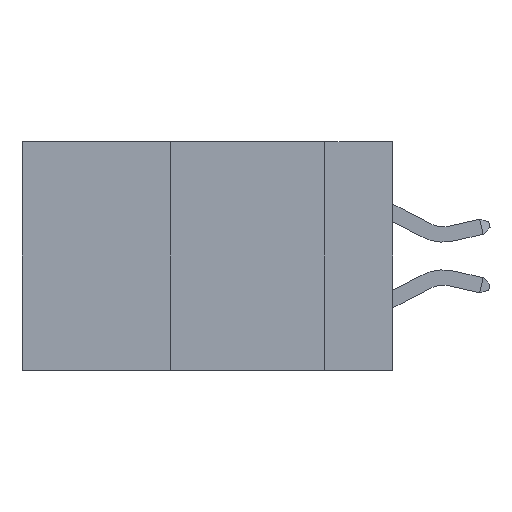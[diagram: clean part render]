
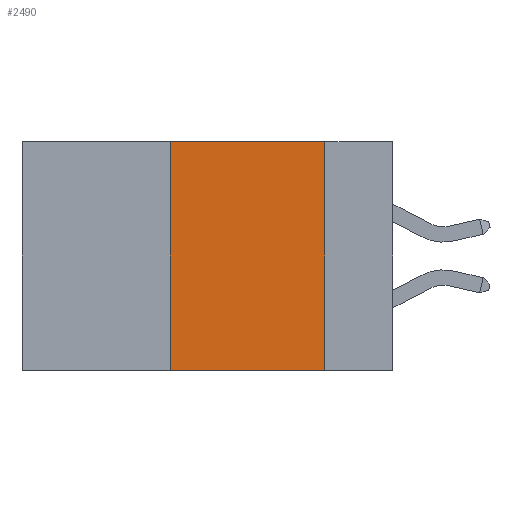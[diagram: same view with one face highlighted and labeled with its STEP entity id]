
A CAD part, left-side view. The second image highlights one B-rep face of the part: STEP entity #2490.
In plain terms, the highlighted planar face has unit normal (-1, 0, 0).
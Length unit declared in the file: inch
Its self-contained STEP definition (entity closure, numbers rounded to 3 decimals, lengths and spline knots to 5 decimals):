
#226 = ORIENTED_EDGE ( 'NONE', *, *, #5466, .F. ) ;
#1595 = VERTEX_POINT ( 'NONE', #4793 ) ;
#1841 = CARTESIAN_POINT ( 'NONE',  ( 0., 0.6, -0.37 ) ) ;
#2490 = ADVANCED_FACE ( 'NONE', ( #16931 ), #11524, .F. ) ;
#2787 = EDGE_LOOP ( 'NONE', ( #31848, #226, #22144, #26153 ) ) ;
#4539 = LINE ( 'NONE', #15166, #14033 ) ;
#4793 = CARTESIAN_POINT ( 'NONE',  ( 0., 0.11, -0.37 ) ) ;
#5466 = EDGE_CURVE ( 'NONE', #10425, #24842, #10987, .T. ) ;
#7572 = DIRECTION ( 'NONE',  ( 0., -1., 0. ) ) ;
#7695 = DIRECTION ( 'NONE',  ( 0., -1., 0. ) ) ;
#8708 = VECTOR ( 'NONE', #33378, 39.37008 ) ;
#9865 = CARTESIAN_POINT ( 'NONE',  ( 0., 0.11, 0. ) ) ;
#10425 = VERTEX_POINT ( 'NONE', #34082 ) ;
#10657 = VECTOR ( 'NONE', #7572, 39.37008 ) ;
#10987 = LINE ( 'NONE', #18673, #29775 ) ;
#11524 = PLANE ( 'NONE',  #22642 ) ;
#11632 = CARTESIAN_POINT ( 'NONE',  ( 0., 0.36, -0.37 ) ) ;
#13168 = EDGE_CURVE ( 'NONE', #21010, #10425, #4539, .T. ) ;
#13965 = DIRECTION ( 'NONE',  ( 0., 0., -1. ) ) ;
#14033 = VECTOR ( 'NONE', #25783, 39.37008 ) ;
#15166 = CARTESIAN_POINT ( 'NONE',  ( 0., 0.36, 0. ) ) ;
#15180 = CARTESIAN_POINT ( 'NONE',  ( 0., 0.11, 0. ) ) ;
#16761 = DIRECTION ( 'NONE',  ( 1., 0., 0. ) ) ;
#16931 = FACE_OUTER_BOUND ( 'NONE', #2787, .T. ) ;
#18673 = CARTESIAN_POINT ( 'NONE',  ( 0., 0.6, 0. ) ) ;
#21010 = VERTEX_POINT ( 'NONE', #11632 ) ;
#21615 = EDGE_CURVE ( 'NONE', #21010, #1595, #31439, .T. ) ;
#22144 = ORIENTED_EDGE ( 'NONE', *, *, #13168, .F. ) ;
#22642 = AXIS2_PLACEMENT_3D ( 'NONE', #24610, #16761, #13965 ) ;
#24610 = CARTESIAN_POINT ( 'NONE',  ( 0., 0.6, 0. ) ) ;
#24842 = VERTEX_POINT ( 'NONE', #15180 ) ;
#25783 = DIRECTION ( 'NONE',  ( 0., 0., 1. ) ) ;
#26153 = ORIENTED_EDGE ( 'NONE', *, *, #21615, .T. ) ;
#26996 = EDGE_CURVE ( 'NONE', #24842, #1595, #33549, .T. ) ;
#29775 = VECTOR ( 'NONE', #7695, 39.37008 ) ;
#31439 = LINE ( 'NONE', #1841, #10657 ) ;
#31848 = ORIENTED_EDGE ( 'NONE', *, *, #26996, .F. ) ;
#33378 = DIRECTION ( 'NONE',  ( 0., 0., -1. ) ) ;
#33549 = LINE ( 'NONE', #9865, #8708 ) ;
#34082 = CARTESIAN_POINT ( 'NONE',  ( 0., 0.36, 0. ) ) ;
